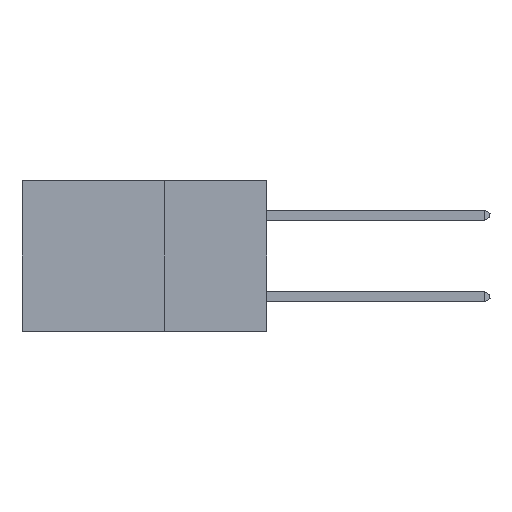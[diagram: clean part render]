
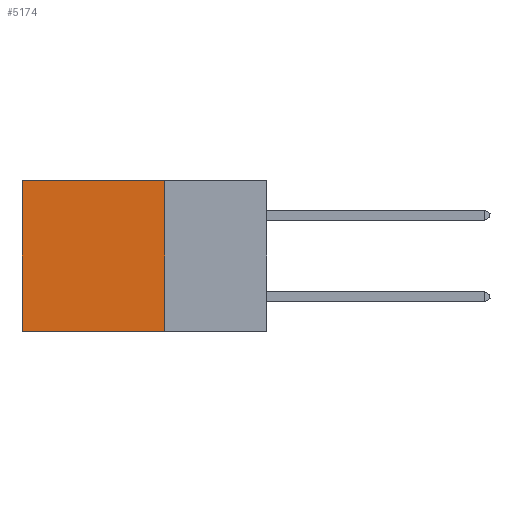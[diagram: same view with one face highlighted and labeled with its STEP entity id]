
A CAD part, left-side view. The second image highlights one B-rep face of the part: STEP entity #5174.
In plain terms, the highlighted planar face has unit normal (-1, 0, 0).
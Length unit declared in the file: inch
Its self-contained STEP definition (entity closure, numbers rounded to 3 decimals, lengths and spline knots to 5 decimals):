
#281 = DIRECTION ( 'NONE',  ( 0., 0., -1. ) ) ;
#662 = CARTESIAN_POINT ( 'NONE',  ( 0.2875, 0.25, 0. ) ) ;
#1643 = CARTESIAN_POINT ( 'NONE',  ( 0.2875, 0.6, 0. ) ) ;
#2075 = DIRECTION ( 'NONE',  ( 1., 0., 0. ) ) ;
#2392 = DIRECTION ( 'NONE',  ( 0., 1., 0. ) ) ;
#2414 = CARTESIAN_POINT ( 'NONE',  ( 0.2875, 0.25, 0. ) ) ;
#3325 = EDGE_CURVE ( 'NONE', #17142, #4745, #17526, .T. ) ;
#3454 = CARTESIAN_POINT ( 'NONE',  ( 0.2875, 0.6, -0.37 ) ) ;
#3841 = AXIS2_PLACEMENT_3D ( 'NONE', #10164, #2075, #13384 ) ;
#4038 = ORIENTED_EDGE ( 'NONE', *, *, #15101, .T. ) ;
#4593 = EDGE_LOOP ( 'NONE', ( #4038, #19923, #6590, #19632 ) ) ;
#4745 = VERTEX_POINT ( 'NONE', #3454 ) ;
#4954 = LINE ( 'NONE', #662, #13050 ) ;
#5032 = LINE ( 'NONE', #19413, #13125 ) ;
#5174 = ADVANCED_FACE ( 'NONE', ( #15977 ), #19488, .F. ) ;
#5976 = LINE ( 'NONE', #1643, #18077 ) ;
#6590 = ORIENTED_EDGE ( 'NONE', *, *, #8958, .F. ) ;
#8958 = EDGE_CURVE ( 'NONE', #12856, #17142, #5032, .T. ) ;
#9540 = VERTEX_POINT ( 'NONE', #11517 ) ;
#10164 = CARTESIAN_POINT ( 'NONE',  ( 0.2875, 0.25, 0. ) ) ;
#10637 = DIRECTION ( 'NONE',  ( 0., 1., 0. ) ) ;
#10863 = CARTESIAN_POINT ( 'NONE',  ( 0.2875, 0.25, -0.37 ) ) ;
#11481 = EDGE_CURVE ( 'NONE', #12856, #9540, #4954, .T. ) ;
#11517 = CARTESIAN_POINT ( 'NONE',  ( 0.2875, 0.6, 0. ) ) ;
#11662 = CARTESIAN_POINT ( 'NONE',  ( 0.2875, 0.25, -0.37 ) ) ;
#12856 = VERTEX_POINT ( 'NONE', #2414 ) ;
#13050 = VECTOR ( 'NONE', #2392, 39.37008 ) ;
#13125 = VECTOR ( 'NONE', #281, 39.37008 ) ;
#13384 = DIRECTION ( 'NONE',  ( 0., 0., -1. ) ) ;
#15101 = EDGE_CURVE ( 'NONE', #9540, #4745, #5976, .T. ) ;
#15923 = DIRECTION ( 'NONE',  ( 0., 0., -1. ) ) ;
#15977 = FACE_OUTER_BOUND ( 'NONE', #4593, .T. ) ;
#17050 = VECTOR ( 'NONE', #10637, 39.37008 ) ;
#17142 = VERTEX_POINT ( 'NONE', #11662 ) ;
#17526 = LINE ( 'NONE', #10863, #17050 ) ;
#18077 = VECTOR ( 'NONE', #15923, 39.37008 ) ;
#19413 = CARTESIAN_POINT ( 'NONE',  ( 0.2875, 0.25, 0. ) ) ;
#19488 = PLANE ( 'NONE',  #3841 ) ;
#19632 = ORIENTED_EDGE ( 'NONE', *, *, #11481, .T. ) ;
#19923 = ORIENTED_EDGE ( 'NONE', *, *, #3325, .F. ) ;
